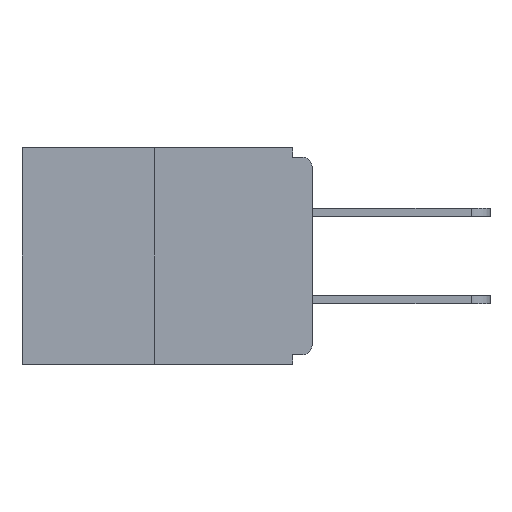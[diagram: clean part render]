
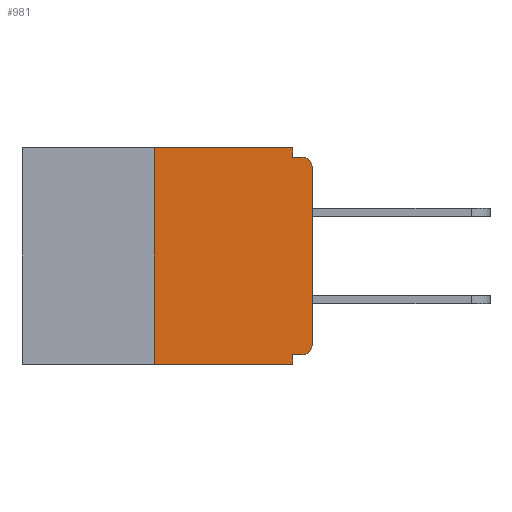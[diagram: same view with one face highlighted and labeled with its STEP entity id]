
A CAD part, left-side view. The second image highlights one B-rep face of the part: STEP entity #981.
In plain terms, the highlighted planar face has unit normal (-1, 0, 0).
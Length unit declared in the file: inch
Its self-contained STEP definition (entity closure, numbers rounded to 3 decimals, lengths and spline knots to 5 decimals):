
#251 = CARTESIAN_POINT ( 'NONE',  ( 0., 0.25, 0. ) ) ;
#981 = ADVANCED_FACE ( 'NONE', ( #4105 ), #13352, .F. ) ;
#1250 = DIRECTION ( 'NONE',  ( 0., -1., 0. ) ) ;
#2386 = VERTEX_POINT ( 'NONE', #13206 ) ;
#2453 = EDGE_CURVE ( 'NONE', #13681, #4919, #17026, .T. ) ;
#2569 = EDGE_CURVE ( 'NONE', #19497, #18395, #19584, .T. ) ;
#2975 = CARTESIAN_POINT ( 'NONE',  ( 0., 0.031, -0.328 ) ) ;
#3198 = CARTESIAN_POINT ( 'NONE',  ( 0., 0.015, -0.03 ) ) ;
#3279 = DIRECTION ( 'NONE',  ( 0., 0., -1. ) ) ;
#3353 = ORIENTED_EDGE ( 'NONE', *, *, #8093, .F. ) ;
#3568 = ORIENTED_EDGE ( 'NONE', *, *, #12867, .T. ) ;
#4105 = FACE_OUTER_BOUND ( 'NONE', #4292, .T. ) ;
#4292 = EDGE_LOOP ( 'NONE', ( #3353, #15963, #11133, #11181, #12366, #13558, #3568, #10993, #5100, #8469 ) ) ;
#4353 = VECTOR ( 'NONE', #3279, 39.37008 ) ;
#4515 = VERTEX_POINT ( 'NONE', #16088 ) ;
#4563 = VERTEX_POINT ( 'NONE', #6171 ) ;
#4638 = DIRECTION ( 'NONE',  ( 0., 0., -1. ) ) ;
#4641 = CARTESIAN_POINT ( 'NONE',  ( 0., 0.031, -0.343 ) ) ;
#4799 = DIRECTION ( 'NONE',  ( 0., 0., -1. ) ) ;
#4919 = VERTEX_POINT ( 'NONE', #2975 ) ;
#5094 = LINE ( 'NONE', #18649, #12370 ) ;
#5100 = ORIENTED_EDGE ( 'NONE', *, *, #16445, .F. ) ;
#5416 = VERTEX_POINT ( 'NONE', #6421 ) ;
#5480 = DIRECTION ( 'NONE',  ( 1., 0., 0. ) ) ;
#5543 = CARTESIAN_POINT ( 'NONE',  ( 0., 0., -0.03 ) ) ;
#5616 = DIRECTION ( 'NONE',  ( 0., -1., 0. ) ) ;
#5858 = EDGE_CURVE ( 'NONE', #4919, #4515, #18959, .T. ) ;
#6067 = VECTOR ( 'NONE', #10094, 39.37008 ) ;
#6143 = VECTOR ( 'NONE', #14638, 39.37008 ) ;
#6171 = CARTESIAN_POINT ( 'NONE',  ( 0., 0., -0.313 ) ) ;
#6421 = CARTESIAN_POINT ( 'NONE',  ( 0., 0.25, -0.343 ) ) ;
#6501 = CARTESIAN_POINT ( 'NONE',  ( 0., 0.015, -0.328 ) ) ;
#6887 = CARTESIAN_POINT ( 'NONE',  ( 0., 0., -0.328 ) ) ;
#7342 = AXIS2_PLACEMENT_3D ( 'NONE', #16965, #8633, #10333 ) ;
#7663 = AXIS2_PLACEMENT_3D ( 'NONE', #12114, #5480, #8879 ) ;
#7784 = EDGE_CURVE ( 'NONE', #5416, #4515, #5094, .T. ) ;
#7899 = CARTESIAN_POINT ( 'NONE',  ( 0., 0., -0.015 ) ) ;
#8054 = CARTESIAN_POINT ( 'NONE',  ( 0., 0., 0. ) ) ;
#8093 = EDGE_CURVE ( 'NONE', #18883, #19915, #12111, .T. ) ;
#8469 = ORIENTED_EDGE ( 'NONE', *, *, #11081, .F. ) ;
#8633 = DIRECTION ( 'NONE',  ( -1., 0., 0. ) ) ;
#8723 = VECTOR ( 'NONE', #1250, 39.37008 ) ;
#8879 = DIRECTION ( 'NONE',  ( 0., 0., -1. ) ) ;
#9308 = LINE ( 'NONE', #18054, #4353 ) ;
#9504 = LINE ( 'NONE', #8054, #6143 ) ;
#10094 = DIRECTION ( 'NONE',  ( 0., 1., 0. ) ) ;
#10333 = DIRECTION ( 'NONE',  ( 0., 0., -1. ) ) ;
#10826 = CARTESIAN_POINT ( 'NONE',  ( 0., 0.46, 0. ) ) ;
#10993 = ORIENTED_EDGE ( 'NONE', *, *, #2569, .T. ) ;
#11081 = EDGE_CURVE ( 'NONE', #19915, #2386, #9308, .T. ) ;
#11133 = ORIENTED_EDGE ( 'NONE', *, *, #7784, .T. ) ;
#11181 = ORIENTED_EDGE ( 'NONE', *, *, #5858, .F. ) ;
#11327 = LINE ( 'NONE', #13224, #12392 ) ;
#12111 = LINE ( 'NONE', #10826, #16016 ) ;
#12114 = CARTESIAN_POINT ( 'NONE',  ( 0., 0.46, 0. ) ) ;
#12366 = ORIENTED_EDGE ( 'NONE', *, *, #2453, .F. ) ;
#12370 = VECTOR ( 'NONE', #20229, 39.37008 ) ;
#12392 = VECTOR ( 'NONE', #15065, 39.37008 ) ;
#12521 = EDGE_CURVE ( 'NONE', #5416, #18883, #11327, .T. ) ;
#12867 = EDGE_CURVE ( 'NONE', #4563, #19497, #9504, .T. ) ;
#13206 = CARTESIAN_POINT ( 'NONE',  ( 0., 0.031, -0.015 ) ) ;
#13224 = CARTESIAN_POINT ( 'NONE',  ( 0., 0.25, 0. ) ) ;
#13352 = PLANE ( 'NONE',  #7663 ) ;
#13558 = ORIENTED_EDGE ( 'NONE', *, *, #17363, .T. ) ;
#13681 = VERTEX_POINT ( 'NONE', #6501 ) ;
#14191 = CIRCLE ( 'NONE', #7342, 0.015 ) ;
#14532 = AXIS2_PLACEMENT_3D ( 'NONE', #3198, #14549, #4638 ) ;
#14549 = DIRECTION ( 'NONE',  ( -1., 0., 0. ) ) ;
#14638 = DIRECTION ( 'NONE',  ( 0., 0., 1. ) ) ;
#15065 = DIRECTION ( 'NONE',  ( 0., 0., 1. ) ) ;
#15963 = ORIENTED_EDGE ( 'NONE', *, *, #12521, .F. ) ;
#16016 = VECTOR ( 'NONE', #5616, 39.37008 ) ;
#16088 = CARTESIAN_POINT ( 'NONE',  ( 0., 0.031, -0.343 ) ) ;
#16445 = EDGE_CURVE ( 'NONE', #2386, #18395, #16831, .T. ) ;
#16662 = CARTESIAN_POINT ( 'NONE',  ( 0., 0.031, 0. ) ) ;
#16831 = LINE ( 'NONE', #7899, #8723 ) ;
#16965 = CARTESIAN_POINT ( 'NONE',  ( 0., 0.015, -0.313 ) ) ;
#17026 = LINE ( 'NONE', #6887, #6067 ) ;
#17363 = EDGE_CURVE ( 'NONE', #13681, #4563, #14191, .T. ) ;
#17932 = VECTOR ( 'NONE', #4799, 39.37008 ) ;
#18054 = CARTESIAN_POINT ( 'NONE',  ( 0., 0.031, 0. ) ) ;
#18395 = VERTEX_POINT ( 'NONE', #18705 ) ;
#18649 = CARTESIAN_POINT ( 'NONE',  ( 0., 0.46, -0.343 ) ) ;
#18705 = CARTESIAN_POINT ( 'NONE',  ( 0., 0.015, -0.015 ) ) ;
#18883 = VERTEX_POINT ( 'NONE', #251 ) ;
#18959 = LINE ( 'NONE', #4641, #17932 ) ;
#19497 = VERTEX_POINT ( 'NONE', #5543 ) ;
#19584 = CIRCLE ( 'NONE', #14532, 0.015 ) ;
#19915 = VERTEX_POINT ( 'NONE', #16662 ) ;
#20229 = DIRECTION ( 'NONE',  ( 0., -1., 0. ) ) ;
